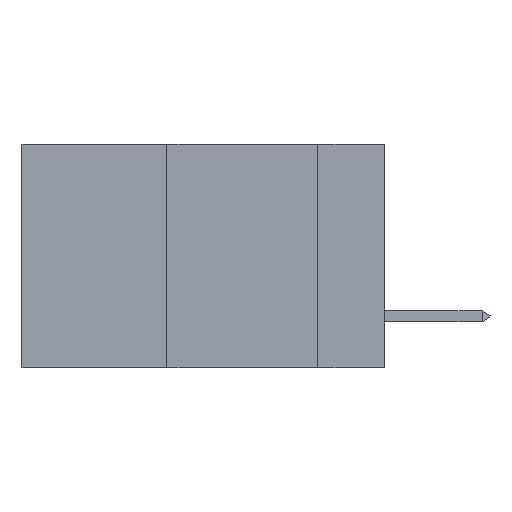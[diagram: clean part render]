
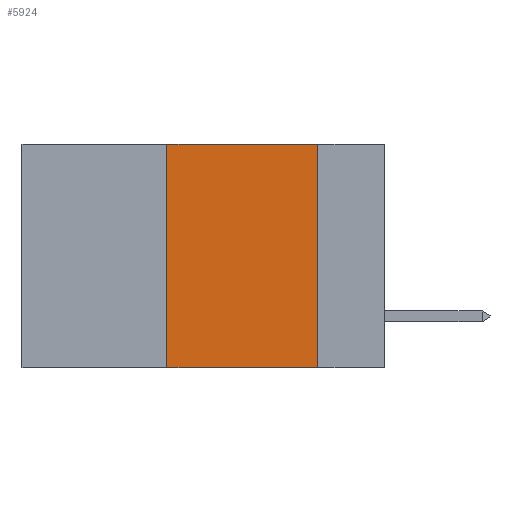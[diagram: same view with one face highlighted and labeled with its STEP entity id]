
A CAD part, left-side view. The second image highlights one B-rep face of the part: STEP entity #5924.
In plain terms, the highlighted planar face has unit normal (-1, 0, 0).
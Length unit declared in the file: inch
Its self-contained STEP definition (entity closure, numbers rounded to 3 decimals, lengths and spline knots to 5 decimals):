
#2134 = EDGE_CURVE ( 'NONE', #19376, #27230, #27643, .T. ) ;
#2971 = CARTESIAN_POINT ( 'NONE',  ( 0., 0.6, 0. ) ) ;
#3246 = LINE ( 'NONE', #12241, #14243 ) ;
#3251 = DIRECTION ( 'NONE',  ( 0., 0., -1. ) ) ;
#4241 = ORIENTED_EDGE ( 'NONE', *, *, #2134, .F. ) ;
#4943 = CARTESIAN_POINT ( 'NONE',  ( 0., 0.11, 0. ) ) ;
#5347 = EDGE_CURVE ( 'NONE', #16154, #27230, #17634, .T. ) ;
#5924 = ADVANCED_FACE ( 'NONE', ( #13754 ), #23370, .F. ) ;
#8457 = CARTESIAN_POINT ( 'NONE',  ( 0., 0.6, -0.37 ) ) ;
#9833 = CARTESIAN_POINT ( 'NONE',  ( 0., 0.11, -0.37 ) ) ;
#10425 = ORIENTED_EDGE ( 'NONE', *, *, #5347, .T. ) ;
#11395 = CARTESIAN_POINT ( 'NONE',  ( 0., 0.36, -0.37 ) ) ;
#12241 = CARTESIAN_POINT ( 'NONE',  ( 0., 0.6, 0. ) ) ;
#13618 = CARTESIAN_POINT ( 'NONE',  ( 0., 0.36, 0. ) ) ;
#13754 = FACE_OUTER_BOUND ( 'NONE', #25793, .T. ) ;
#14180 = DIRECTION ( 'NONE',  ( 0., 0., 1. ) ) ;
#14243 = VECTOR ( 'NONE', #19055, 39.37008 ) ;
#14273 = AXIS2_PLACEMENT_3D ( 'NONE', #2971, #18779, #16539 ) ;
#14439 = VECTOR ( 'NONE', #3251, 39.37008 ) ;
#16154 = VERTEX_POINT ( 'NONE', #11395 ) ;
#16407 = CARTESIAN_POINT ( 'NONE',  ( 0., 0.11, 0. ) ) ;
#16539 = DIRECTION ( 'NONE',  ( 0., 0., -1. ) ) ;
#16855 = EDGE_CURVE ( 'NONE', #16154, #19881, #18628, .T. ) ;
#17634 = LINE ( 'NONE', #8457, #22275 ) ;
#18628 = LINE ( 'NONE', #24991, #23652 ) ;
#18779 = DIRECTION ( 'NONE',  ( 1., 0., 0. ) ) ;
#19055 = DIRECTION ( 'NONE',  ( 0., -1., 0. ) ) ;
#19376 = VERTEX_POINT ( 'NONE', #4943 ) ;
#19881 = VERTEX_POINT ( 'NONE', #13618 ) ;
#22275 = VECTOR ( 'NONE', #26662, 39.37008 ) ;
#23370 = PLANE ( 'NONE',  #14273 ) ;
#23557 = ORIENTED_EDGE ( 'NONE', *, *, #16855, .F. ) ;
#23652 = VECTOR ( 'NONE', #14180, 39.37008 ) ;
#24046 = EDGE_CURVE ( 'NONE', #19881, #19376, #3246, .T. ) ;
#24207 = ORIENTED_EDGE ( 'NONE', *, *, #24046, .F. ) ;
#24991 = CARTESIAN_POINT ( 'NONE',  ( 0., 0.36, 0. ) ) ;
#25793 = EDGE_LOOP ( 'NONE', ( #4241, #24207, #23557, #10425 ) ) ;
#26662 = DIRECTION ( 'NONE',  ( 0., -1., 0. ) ) ;
#27230 = VERTEX_POINT ( 'NONE', #9833 ) ;
#27643 = LINE ( 'NONE', #16407, #14439 ) ;
